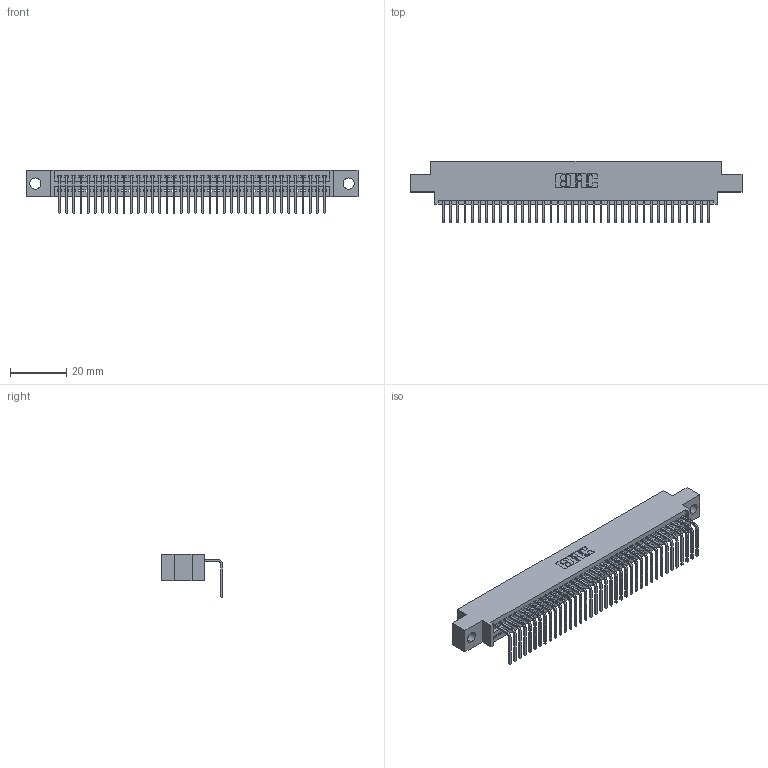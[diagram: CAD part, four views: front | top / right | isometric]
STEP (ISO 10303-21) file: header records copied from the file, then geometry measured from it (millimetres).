
FILE_DESCRIPTION (( 'STEP AP203' ), '1' );
FILE_NAME ('395-038-558-604.STEP', '2021-06-11T14:45:15', ( '' ), ( '' ), 'SwSTEP 2.0', 'SolidWorks 2020', '' );
FILE_SCHEMA (( 'CONFIG_CONTROL_DESIGN' ));
Length unit declared in the file: inch
Products named in the file (3): 345 Part_0.170 Offset - 0.156 Dia-TI; 345-292-001_558 Tail - 2; 395-038-558-604
Assembly tree (39 placements, depth 2):
  395-038-558-604
    345 Part_0.170 Offset - 0.156 Dia-TI
    345-292-001_558 Tail - 2  x38
Bounding box: 117.73 x 21.83 x 15.37 mm (x, y, z)
Volume: 11056.5 mm3; surface area: 15351.7 mm2
Topology: 39 solids, 39 shells, 2424 faces, 7305 edges, 4818 vertices
Faces by surface type: plane 1694, cylinder 730
Entity records: 29773 total; most frequent: CARTESIAN_POINT 5168, ORIENTED_EDGE 5138, DIRECTION 4517, EDGE_CURVE 2569, VECTOR 2285, LINE 2285, VERTEX_POINT 1710, AXIS2_PLACEMENT_3D 1116
